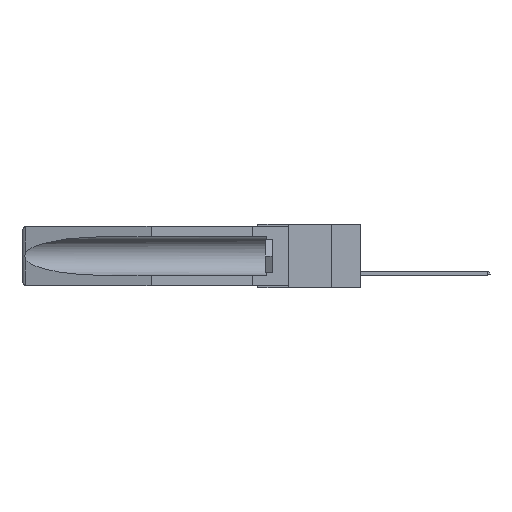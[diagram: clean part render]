
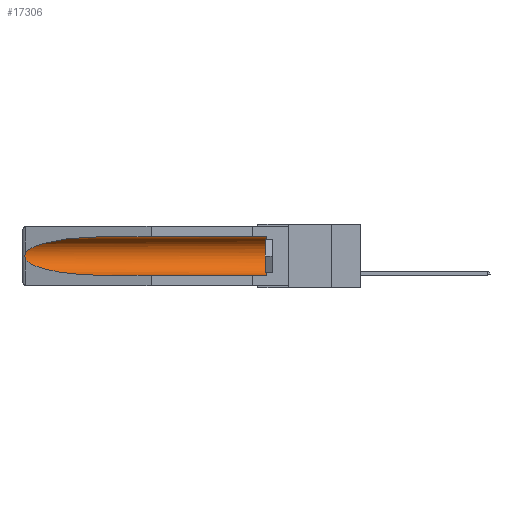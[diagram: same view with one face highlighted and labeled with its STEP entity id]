
A CAD part, left-side view. The second image highlights one B-rep face of the part: STEP entity #17306.
In plain terms, the highlighted cylindrical face has radius 2.857 mm (diameter 5.715 mm), a partial arc.
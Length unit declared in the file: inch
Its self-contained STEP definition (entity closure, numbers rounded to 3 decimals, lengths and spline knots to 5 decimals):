
#1677 = CARTESIAN_POINT ( 'NONE',  ( 0.155, -0.30754, -0.059 ) ) ;
#1697 = CARTESIAN_POINT ( 'NONE',  ( 0.25451, 1.48313, -0.09465 ) ) ;
#1795 = EDGE_CURVE ( 'NONE', #20039, #5546, #14096, .T. ) ;
#1873 = AXIS2_PLACEMENT_3D ( 'NONE', #9790, #15895, #7923 ) ;
#1961 = CARTESIAN_POINT ( 'NONE',  ( 0.26537, 1.52718, -0.19328 ) ) ;
#1992 = ORIENTED_EDGE ( 'NONE', *, *, #4166, .T. ) ;
#2081 = ORIENTED_EDGE ( 'NONE', *, *, #1795, .T. ) ;
#2894 = VECTOR ( 'NONE', #18207, 39.37008 ) ;
#3095 = CARTESIAN_POINT ( 'NONE',  ( 0.26597, 1.52961, -0.15275 ) ) ;
#3530 = FACE_OUTER_BOUND ( 'NONE', #5668, .T. ) ;
#3725 = VERTEX_POINT ( 'NONE', #22021 ) ;
#4166 = EDGE_CURVE ( 'NONE', #5546, #3725, #14033, .T. ) ;
#4902 = CARTESIAN_POINT ( 'NONE',  ( 0.2673, 1.53269, -0.17917 ) ) ;
#5155 = CARTESIAN_POINT ( 'NONE',  ( 0.155, 1.07973, -0.284 ) ) ;
#5530 = ORIENTED_EDGE ( 'NONE', *, *, #11075, .F. ) ;
#5546 = VERTEX_POINT ( 'NONE', #9700 ) ;
#5564 = VECTOR ( 'NONE', #7596, 39.37008 ) ;
#5668 = EDGE_LOOP ( 'NONE', ( #1992, #14194, #21166, #5530, #19274, #2081 ) ) ;
#6920 = CARTESIAN_POINT ( 'NONE',  ( 0.26537, 1.52718, -0.19328 ) ) ;
#7097 = CARTESIAN_POINT ( 'NONE',  ( 0.26654, 1.53092, -0.15636 ) ) ;
#7596 = DIRECTION ( 'NONE',  ( 0., 1., 0. ) ) ;
#7923 = DIRECTION ( 'NONE',  ( 0., 0., 1. ) ) ;
#8869 = CARTESIAN_POINT ( 'NONE',  ( 0.21114, 1.30732, -0.284 ) ) ;
#9548 = CARTESIAN_POINT ( 'NONE',  ( 0.21114, 1.30732, -0.059 ) ) ;
#9700 = CARTESIAN_POINT ( 'NONE',  ( 0.155, 1.07973, -0.059 ) ) ;
#9790 = CARTESIAN_POINT ( 'NONE',  ( 0.155, -0.30754, -0.1715 ) ) ;
#10068 = CYLINDRICAL_SURFACE ( 'NONE', #1873, 0.1125 ) ;
#10089 = CARTESIAN_POINT ( 'NONE',  ( 0.155, -0.30754, -0.284 ) ) ;
#10225 = CARTESIAN_POINT ( 'NONE',  ( 0.155, 0.126, -0.1715 ) ) ;
#11075 = EDGE_CURVE ( 'NONE', #11388, #24183, #19142, .T. ) ;
#11388 = VERTEX_POINT ( 'NONE', #15073 ) ;
#11421 = B_SPLINE_CURVE_WITH_KNOTS ( 'NONE', 3,
 ( #17166, #3095, #7097, #25184, #19172, #21054, #4902, #18823, #18903, #6920 ),
 .UNSPECIFIED., .F., .F.,
 ( 4, 2, 2, 2, 4 ),
 ( 0., 0.00029, 0.00058, 0.00087, 0.00117 ),
 .UNSPECIFIED. ) ;
#11647 = AXIS2_PLACEMENT_3D ( 'NONE', #10225, #18257, #24181 ) ;
#14033 =( BOUNDED_CURVE ( )  B_SPLINE_CURVE ( 3, ( #21474, #9548, #1697, #25248 ),
 .UNSPECIFIED., .F., .T. ) 
 B_SPLINE_CURVE_WITH_KNOTS ( ( 4, 4 ),
 ( 4.71239, 6.08839 ),
 .UNSPECIFIED. ) 
 CURVE ( )  GEOMETRIC_REPRESENTATION_ITEM ( )  RATIONAL_B_SPLINE_CURVE ( ( 1., 0.848, 0.848, 1. ) ) 
 REPRESENTATION_ITEM ( '' )  );
#14096 = LINE ( 'NONE', #1677, #5564 ) ;
#14194 = ORIENTED_EDGE ( 'NONE', *, *, #23489, .T. ) ;
#14663 = EDGE_CURVE ( 'NONE', #18914, #24183, #19942, .T. ) ;
#15073 = CARTESIAN_POINT ( 'NONE',  ( 0.155, 0.126, -0.284 ) ) ;
#15895 = DIRECTION ( 'NONE',  ( 0., 1., 0. ) ) ;
#17166 = CARTESIAN_POINT ( 'NONE',  ( 0.26537, 1.52718, -0.14972 ) ) ;
#17306 = ADVANCED_FACE ( 'NONE', ( #3530 ), #10068, .F. ) ;
#18207 = DIRECTION ( 'NONE',  ( 0., 1., 0. ) ) ;
#18257 = DIRECTION ( 'NONE',  ( 0., -1., 0. ) ) ;
#18823 = CARTESIAN_POINT ( 'NONE',  ( 0.26655, 1.53094, -0.18657 ) ) ;
#18903 = CARTESIAN_POINT ( 'NONE',  ( 0.26597, 1.5296, -0.19026 ) ) ;
#18914 = VERTEX_POINT ( 'NONE', #1961 ) ;
#19142 = LINE ( 'NONE', #10089, #2894 ) ;
#19172 = CARTESIAN_POINT ( 'NONE',  ( 0.2675, 1.53308, -0.16763 ) ) ;
#19274 = ORIENTED_EDGE ( 'NONE', *, *, #22568, .T. ) ;
#19942 =( BOUNDED_CURVE ( )  B_SPLINE_CURVE ( 3, ( #22988, #25095, #8869, #22810 ),
 .UNSPECIFIED., .F., .F. ) 
 B_SPLINE_CURVE_WITH_KNOTS ( ( 4, 4 ),
 ( 0.1948, 1.5708 ),
 .UNSPECIFIED. ) 
 CURVE ( )  GEOMETRIC_REPRESENTATION_ITEM ( )  RATIONAL_B_SPLINE_CURVE ( ( 1., 0.848, 0.848, 1. ) ) 
 REPRESENTATION_ITEM ( '' )  );
#20039 = VERTEX_POINT ( 'NONE', #21169 ) ;
#21054 = CARTESIAN_POINT ( 'NONE',  ( 0.2675, 1.53308, -0.17534 ) ) ;
#21166 = ORIENTED_EDGE ( 'NONE', *, *, #14663, .T. ) ;
#21169 = CARTESIAN_POINT ( 'NONE',  ( 0.155, 0.126, -0.059 ) ) ;
#21474 = CARTESIAN_POINT ( 'NONE',  ( 0.155, 1.07973, -0.059 ) ) ;
#22021 = CARTESIAN_POINT ( 'NONE',  ( 0.26537, 1.52718, -0.14972 ) ) ;
#22568 = EDGE_CURVE ( 'NONE', #11388, #20039, #23300, .T. ) ;
#22810 = CARTESIAN_POINT ( 'NONE',  ( 0.155, 1.07973, -0.284 ) ) ;
#22988 = CARTESIAN_POINT ( 'NONE',  ( 0.26537, 1.52718, -0.19328 ) ) ;
#23300 = CIRCLE ( 'NONE', #11647, 0.1125 ) ;
#23489 = EDGE_CURVE ( 'NONE', #3725, #18914, #11421, .T. ) ;
#24181 = DIRECTION ( 'NONE',  ( 0., 0., 1. ) ) ;
#24183 = VERTEX_POINT ( 'NONE', #5155 ) ;
#25095 = CARTESIAN_POINT ( 'NONE',  ( 0.25451, 1.48313, -0.24835 ) ) ;
#25184 = CARTESIAN_POINT ( 'NONE',  ( 0.2673, 1.5327, -0.16383 ) ) ;
#25248 = CARTESIAN_POINT ( 'NONE',  ( 0.26537, 1.52718, -0.14972 ) ) ;
